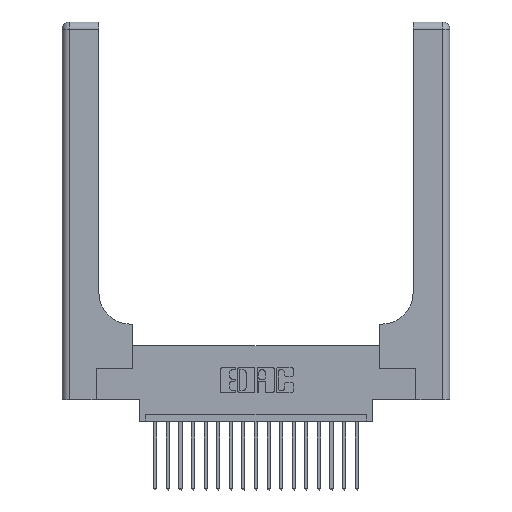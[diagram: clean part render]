
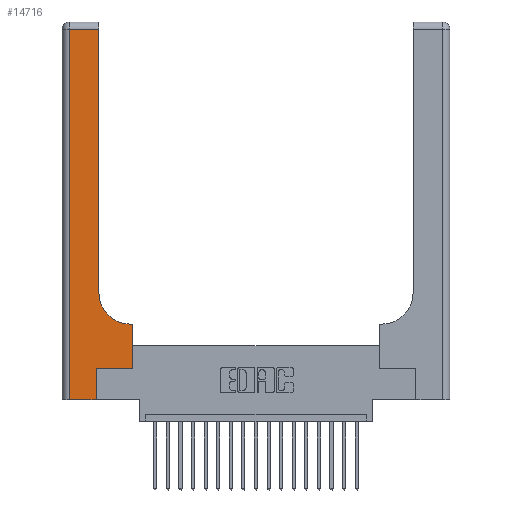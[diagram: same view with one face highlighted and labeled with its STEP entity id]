
A CAD part, top view. The second image highlights one B-rep face of the part: STEP entity #14716.
In plain terms, the highlighted planar face has unit normal (0, 0, 1).
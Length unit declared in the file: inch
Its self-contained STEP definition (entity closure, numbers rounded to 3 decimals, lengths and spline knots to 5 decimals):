
#440 = DIRECTION ( 'NONE',  ( 1., 0., 0. ) ) ;
#604 = DIRECTION ( 'NONE',  ( 1., 0., 0. ) ) ;
#880 = EDGE_CURVE ( 'NONE', #4291, #5516, #18530, .T. ) ;
#942 = VECTOR ( 'NONE', #440, 39.37008 ) ;
#994 = PLANE ( 'NONE',  #5626 ) ;
#1184 = LINE ( 'NONE', #6389, #5158 ) ;
#1533 = EDGE_LOOP ( 'NONE', ( #19410, #11744, #2802, #8453, #11895, #17719, #6130, #17188, #19556 ) ) ;
#1598 = DIRECTION ( 'NONE',  ( 0., 1., 0. ) ) ;
#2435 = CARTESIAN_POINT ( 'NONE',  ( 0.269, 0.25, 0.37 ) ) ;
#2673 = CARTESIAN_POINT ( 'NONE',  ( 0., 2.94, 0.37 ) ) ;
#2731 = EDGE_CURVE ( 'NONE', #5516, #13681, #18482, .T. ) ;
#2802 = ORIENTED_EDGE ( 'NONE', *, *, #11470, .T. ) ;
#2968 = CARTESIAN_POINT ( 'NONE',  ( 0.2915, 2.94, 0.37 ) ) ;
#3523 = DIRECTION ( 'NONE',  ( 0., 1., 0. ) ) ;
#4004 = VECTOR ( 'NONE', #16131, 39.37008 ) ;
#4093 = CARTESIAN_POINT ( 'NONE',  ( 0., 3., 0.37 ) ) ;
#4291 = VERTEX_POINT ( 'NONE', #19815 ) ;
#4865 = AXIS2_PLACEMENT_3D ( 'NONE', #7128, #9017, #604 ) ;
#5003 = CARTESIAN_POINT ( 'NONE',  ( 0.5585, 0.25, 0.37 ) ) ;
#5158 = VECTOR ( 'NONE', #6611, 39.37008 ) ;
#5296 = EDGE_CURVE ( 'NONE', #6568, #16774, #9843, .T. ) ;
#5516 = VERTEX_POINT ( 'NONE', #11931 ) ;
#5626 = AXIS2_PLACEMENT_3D ( 'NONE', #4093, #12654, #10708 ) ;
#6130 = ORIENTED_EDGE ( 'NONE', *, *, #18106, .T. ) ;
#6389 = CARTESIAN_POINT ( 'NONE',  ( 0., 0., 0.37 ) ) ;
#6568 = VERTEX_POINT ( 'NONE', #2435 ) ;
#6611 = DIRECTION ( 'NONE',  ( 1., 0., 0. ) ) ;
#6870 = LINE ( 'NONE', #2673, #9698 ) ;
#7118 = CARTESIAN_POINT ( 'NONE',  ( 0.269, 0.25, 0.37 ) ) ;
#7128 = CARTESIAN_POINT ( 'NONE',  ( 0.5415, 0.85, 0.37 ) ) ;
#7797 = CARTESIAN_POINT ( 'NONE',  ( 0.5585, 0.25, 0.37 ) ) ;
#7937 = EDGE_CURVE ( 'NONE', #13681, #8137, #9069, .T. ) ;
#8137 = VERTEX_POINT ( 'NONE', #2968 ) ;
#8453 = ORIENTED_EDGE ( 'NONE', *, *, #8711, .T. ) ;
#8711 = EDGE_CURVE ( 'NONE', #17065, #18123, #1184, .T. ) ;
#8965 = CARTESIAN_POINT ( 'NONE',  ( 0.269, 0., 0.37 ) ) ;
#9017 = DIRECTION ( 'NONE',  ( 0., 0., -1. ) ) ;
#9069 = LINE ( 'NONE', #15236, #17341 ) ;
#9527 = CARTESIAN_POINT ( 'NONE',  ( 0.2915, 0.85, 0.37 ) ) ;
#9698 = VECTOR ( 'NONE', #10836, 39.37008 ) ;
#9843 = LINE ( 'NONE', #7118, #942 ) ;
#10606 = CARTESIAN_POINT ( 'NONE',  ( 0.06, 3., 0.37 ) ) ;
#10708 = DIRECTION ( 'NONE',  ( -1., 0., 0. ) ) ;
#10836 = DIRECTION ( 'NONE',  ( -1., 0., 0. ) ) ;
#11470 = EDGE_CURVE ( 'NONE', #17169, #17065, #12570, .T. ) ;
#11744 = ORIENTED_EDGE ( 'NONE', *, *, #14717, .T. ) ;
#11895 = ORIENTED_EDGE ( 'NONE', *, *, #19345, .T. ) ;
#11931 = CARTESIAN_POINT ( 'NONE',  ( 0.5415, 0.6, 0.37 ) ) ;
#12305 = FACE_OUTER_BOUND ( 'NONE', #1533, .T. ) ;
#12570 = LINE ( 'NONE', #10606, #19814 ) ;
#12654 = DIRECTION ( 'NONE',  ( 0., 0., -1. ) ) ;
#13681 = VERTEX_POINT ( 'NONE', #9527 ) ;
#14534 = CARTESIAN_POINT ( 'NONE',  ( 0.2915, 0.6, 0.37 ) ) ;
#14716 = ADVANCED_FACE ( 'NONE', ( #12305 ), #994, .F. ) ;
#14717 = EDGE_CURVE ( 'NONE', #8137, #17169, #6870, .T. ) ;
#15236 = CARTESIAN_POINT ( 'NONE',  ( 0.2915, 3., 0.37 ) ) ;
#15595 = VECTOR ( 'NONE', #17680, 39.37008 ) ;
#15618 = DIRECTION ( 'NONE',  ( 0., -1., 0. ) ) ;
#16131 = DIRECTION ( 'NONE',  ( -1., 0., 0. ) ) ;
#16326 = LINE ( 'NONE', #5003, #17112 ) ;
#16774 = VERTEX_POINT ( 'NONE', #7797 ) ;
#17065 = VERTEX_POINT ( 'NONE', #20214 ) ;
#17112 = VECTOR ( 'NONE', #1598, 39.37008 ) ;
#17169 = VERTEX_POINT ( 'NONE', #20835 ) ;
#17188 = ORIENTED_EDGE ( 'NONE', *, *, #880, .T. ) ;
#17341 = VECTOR ( 'NONE', #3523, 39.37008 ) ;
#17680 = DIRECTION ( 'NONE',  ( 0., 1., 0. ) ) ;
#17719 = ORIENTED_EDGE ( 'NONE', *, *, #5296, .T. ) ;
#18106 = EDGE_CURVE ( 'NONE', #16774, #4291, #16326, .T. ) ;
#18123 = VERTEX_POINT ( 'NONE', #20449 ) ;
#18482 = CIRCLE ( 'NONE', #4865, 0.25 ) ;
#18530 = LINE ( 'NONE', #14534, #4004 ) ;
#19345 = EDGE_CURVE ( 'NONE', #18123, #6568, #19969, .T. ) ;
#19410 = ORIENTED_EDGE ( 'NONE', *, *, #7937, .T. ) ;
#19556 = ORIENTED_EDGE ( 'NONE', *, *, #2731, .T. ) ;
#19814 = VECTOR ( 'NONE', #15618, 39.37008 ) ;
#19815 = CARTESIAN_POINT ( 'NONE',  ( 0.5585, 0.6, 0.37 ) ) ;
#19969 = LINE ( 'NONE', #8965, #15595 ) ;
#20214 = CARTESIAN_POINT ( 'NONE',  ( 0.06, 0., 0.37 ) ) ;
#20449 = CARTESIAN_POINT ( 'NONE',  ( 0.269, 0., 0.37 ) ) ;
#20835 = CARTESIAN_POINT ( 'NONE',  ( 0.06, 2.94, 0.37 ) ) ;
